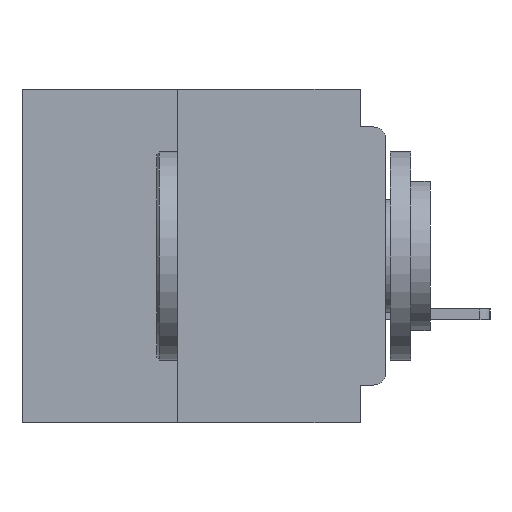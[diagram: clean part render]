
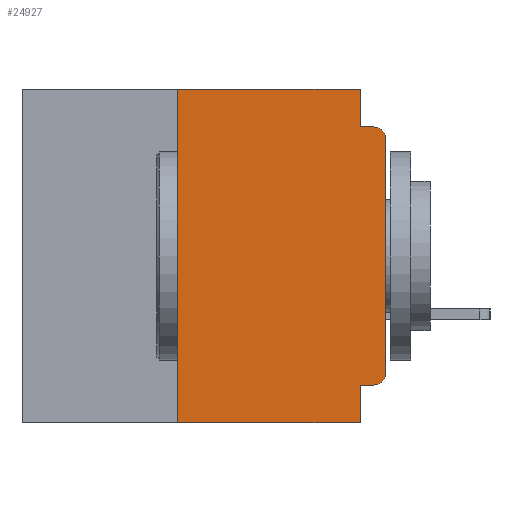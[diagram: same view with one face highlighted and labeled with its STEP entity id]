
A CAD part, left-side view. The second image highlights one B-rep face of the part: STEP entity #24927.
In plain terms, the highlighted planar face has unit normal (-1, 0, 0).
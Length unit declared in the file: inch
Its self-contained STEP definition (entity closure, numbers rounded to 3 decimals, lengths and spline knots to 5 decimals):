
#25 = CARTESIAN_POINT ( 'NONE',  ( 0., 0.031, -0.4 ) ) ;
#477 = EDGE_CURVE ( 'NONE', #42407, #30764, #5272, .T. ) ;
#710 = ORIENTED_EDGE ( 'NONE', *, *, #29747, .T. ) ;
#816 = CARTESIAN_POINT ( 'NONE',  ( 0., 0.437, -0.4 ) ) ;
#1371 = EDGE_CURVE ( 'NONE', #20383, #42407, #45631, .T. ) ;
#1873 = VERTEX_POINT ( 'NONE', #25109 ) ;
#3715 = CARTESIAN_POINT ( 'NONE',  ( 0., 0.015, -0.34 ) ) ;
#4328 = ORIENTED_EDGE ( 'NONE', *, *, #477, .F. ) ;
#4372 = DIRECTION ( 'NONE',  ( 0., 0., -1. ) ) ;
#4450 = CARTESIAN_POINT ( 'NONE',  ( 0., 0.437, 0. ) ) ;
#4612 = CARTESIAN_POINT ( 'NONE',  ( 0., 0.25, -0.4 ) ) ;
#5244 = LINE ( 'NONE', #41355, #15454 ) ;
#5272 = LINE ( 'NONE', #4450, #35765 ) ;
#5383 = DIRECTION ( 'NONE',  ( 0., -1., 0. ) ) ;
#6376 = EDGE_LOOP ( 'NONE', ( #710, #41989, #7529, #36752, #4328, #47267, #8173, #45478, #46885, #34880 ) ) ;
#7529 = ORIENTED_EDGE ( 'NONE', *, *, #22021, .F. ) ;
#8100 = DIRECTION ( 'NONE',  ( 0., 0., -1. ) ) ;
#8173 = ORIENTED_EDGE ( 'NONE', *, *, #41384, .T. ) ;
#8316 = EDGE_CURVE ( 'NONE', #50469, #54930, #15348, .T. ) ;
#8838 = LINE ( 'NONE', #18100, #50508 ) ;
#10758 = DIRECTION ( 'NONE',  ( 0., 0., 1. ) ) ;
#11005 = CARTESIAN_POINT ( 'NONE',  ( 0., 0.015, -0.355 ) ) ;
#11181 = DIRECTION ( 'NONE',  ( 0., 0., -1. ) ) ;
#12140 = LINE ( 'NONE', #32363, #22296 ) ;
#14189 = CARTESIAN_POINT ( 'NONE',  ( 0., 0.015, -0.06 ) ) ;
#14205 = AXIS2_PLACEMENT_3D ( 'NONE', #14189, #44300, #18517 ) ;
#15283 = EDGE_CURVE ( 'NONE', #42243, #1873, #8838, .T. ) ;
#15348 = CIRCLE ( 'NONE', #14205, 0.015 ) ;
#15454 = VECTOR ( 'NONE', #11181, 39.37008 ) ;
#16674 = CARTESIAN_POINT ( 'NONE',  ( 0., 0.25, 0. ) ) ;
#18100 = CARTESIAN_POINT ( 'NONE',  ( 0., 0., -0.355 ) ) ;
#18517 = DIRECTION ( 'NONE',  ( 0., 0., -1. ) ) ;
#18592 = VERTEX_POINT ( 'NONE', #51621 ) ;
#19917 = CIRCLE ( 'NONE', #47974, 0.015 ) ;
#20077 = CARTESIAN_POINT ( 'NONE',  ( 0., 0.031, -0.045 ) ) ;
#20223 = CARTESIAN_POINT ( 'NONE',  ( 0., 0.437, 0. ) ) ;
#20383 = VERTEX_POINT ( 'NONE', #4612 ) ;
#22021 = EDGE_CURVE ( 'NONE', #29476, #54930, #29837, .T. ) ;
#22296 = VECTOR ( 'NONE', #10758, 39.37008 ) ;
#22630 = DIRECTION ( 'NONE',  ( 0., 1., 0. ) ) ;
#24601 = DIRECTION ( 'NONE',  ( 0., 0., -1. ) ) ;
#24927 = ADVANCED_FACE ( 'NONE', ( #40874 ), #41695, .F. ) ;
#25055 = EDGE_CURVE ( 'NONE', #42243, #18592, #19917, .T. ) ;
#25109 = CARTESIAN_POINT ( 'NONE',  ( 0., 0.031, -0.355 ) ) ;
#25522 = LINE ( 'NONE', #25, #46965 ) ;
#28589 = VERTEX_POINT ( 'NONE', #48334 ) ;
#29476 = VERTEX_POINT ( 'NONE', #20077 ) ;
#29747 = EDGE_CURVE ( 'NONE', #18592, #50469, #12140, .T. ) ;
#29837 = LINE ( 'NONE', #34884, #49839 ) ;
#30744 = CARTESIAN_POINT ( 'NONE',  ( 0., 0.031, 0. ) ) ;
#30764 = VERTEX_POINT ( 'NONE', #30744 ) ;
#30801 = CARTESIAN_POINT ( 'NONE',  ( 0., 0., -0.06 ) ) ;
#32363 = CARTESIAN_POINT ( 'NONE',  ( 0., 0., 0. ) ) ;
#34038 = DIRECTION ( 'NONE',  ( -1., 0., 0. ) ) ;
#34880 = ORIENTED_EDGE ( 'NONE', *, *, #25055, .T. ) ;
#34884 = CARTESIAN_POINT ( 'NONE',  ( 0., 0., -0.045 ) ) ;
#35765 = VECTOR ( 'NONE', #46390, 39.37008 ) ;
#36591 = AXIS2_PLACEMENT_3D ( 'NONE', #20223, #50214, #24601 ) ;
#36752 = ORIENTED_EDGE ( 'NONE', *, *, #49536, .F. ) ;
#39727 = LINE ( 'NONE', #816, #48338 ) ;
#40874 = FACE_OUTER_BOUND ( 'NONE', #6376, .T. ) ;
#41355 = CARTESIAN_POINT ( 'NONE',  ( 0., 0.031, 0. ) ) ;
#41384 = EDGE_CURVE ( 'NONE', #20383, #28589, #39727, .T. ) ;
#41695 = PLANE ( 'NONE',  #36591 ) ;
#41872 = EDGE_CURVE ( 'NONE', #1873, #28589, #25522, .T. ) ;
#41989 = ORIENTED_EDGE ( 'NONE', *, *, #8316, .T. ) ;
#42243 = VERTEX_POINT ( 'NONE', #11005 ) ;
#42407 = VERTEX_POINT ( 'NONE', #16674 ) ;
#44300 = DIRECTION ( 'NONE',  ( -1., 0., 0. ) ) ;
#45478 = ORIENTED_EDGE ( 'NONE', *, *, #41872, .F. ) ;
#45631 = LINE ( 'NONE', #46431, #55570 ) ;
#46300 = DIRECTION ( 'NONE',  ( 0., 0., 1. ) ) ;
#46390 = DIRECTION ( 'NONE',  ( 0., -1., 0. ) ) ;
#46431 = CARTESIAN_POINT ( 'NONE',  ( 0., 0.25, -0.4 ) ) ;
#46885 = ORIENTED_EDGE ( 'NONE', *, *, #15283, .F. ) ;
#46965 = VECTOR ( 'NONE', #4372, 39.37008 ) ;
#47267 = ORIENTED_EDGE ( 'NONE', *, *, #1371, .F. ) ;
#47713 = DIRECTION ( 'NONE',  ( 0., -1., 0. ) ) ;
#47974 = AXIS2_PLACEMENT_3D ( 'NONE', #3715, #34038, #8100 ) ;
#48334 = CARTESIAN_POINT ( 'NONE',  ( 0., 0.031, -0.4 ) ) ;
#48338 = VECTOR ( 'NONE', #5383, 39.37008 ) ;
#49536 = EDGE_CURVE ( 'NONE', #30764, #29476, #5244, .T. ) ;
#49839 = VECTOR ( 'NONE', #47713, 39.37008 ) ;
#50214 = DIRECTION ( 'NONE',  ( 1., 0., 0. ) ) ;
#50469 = VERTEX_POINT ( 'NONE', #30801 ) ;
#50508 = VECTOR ( 'NONE', #22630, 39.37008 ) ;
#51318 = CARTESIAN_POINT ( 'NONE',  ( 0., 0.015, -0.045 ) ) ;
#51621 = CARTESIAN_POINT ( 'NONE',  ( 0., 0., -0.34 ) ) ;
#54930 = VERTEX_POINT ( 'NONE', #51318 ) ;
#55570 = VECTOR ( 'NONE', #46300, 39.37008 ) ;
